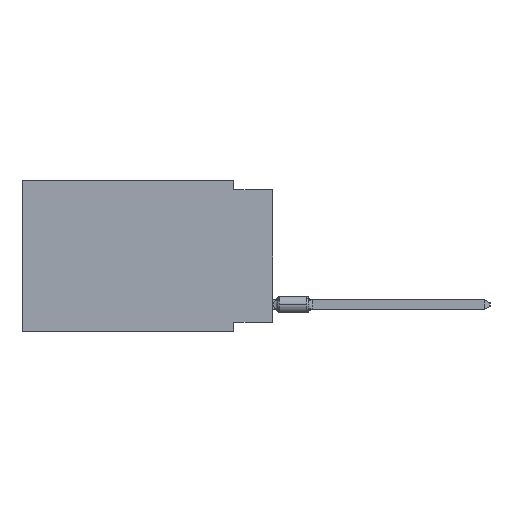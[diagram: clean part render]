
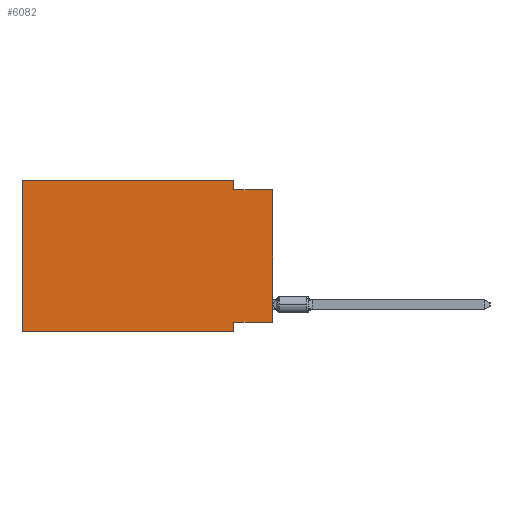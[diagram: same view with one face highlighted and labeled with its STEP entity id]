
A CAD part, left-side view. The second image highlights one B-rep face of the part: STEP entity #6082.
In plain terms, the highlighted planar face has unit normal (-1, 0, 0).
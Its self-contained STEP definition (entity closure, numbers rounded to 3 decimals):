
#603 = PLANE ( 'NONE',  #39979 ) ;
#1927 = LINE ( 'NONE', #6170, #13339 ) ;
#2528 = ORIENTED_EDGE ( 'NONE', *, *, #39677, .F. ) ;
#4096 = VECTOR ( 'NONE', #33010, 1000. ) ;
#4972 = LINE ( 'NONE', #29674, #46777 ) ;
#5116 = CARTESIAN_POINT ( 'NONE',  ( 0., 16.383, 0. ) ) ;
#5602 = ORIENTED_EDGE ( 'NONE', *, *, #21549, .F. ) ;
#6082 = ADVANCED_FACE ( 'NONE', ( #37013 ), #603, .F. ) ;
#6170 = CARTESIAN_POINT ( 'NONE',  ( 0., 0., -0.635 ) ) ;
#6790 = LINE ( 'NONE', #30448, #42864 ) ;
#8175 = EDGE_CURVE ( 'NONE', #9592, #27998, #50146, .T. ) ;
#9592 = VERTEX_POINT ( 'NONE', #29975 ) ;
#10128 = LINE ( 'NONE', #50221, #23848 ) ;
#10316 = DIRECTION ( 'NONE',  ( 0., -1., 0. ) ) ;
#10340 = VERTEX_POINT ( 'NONE', #44719 ) ;
#10588 = DIRECTION ( 'NONE',  ( 0., 0., -1. ) ) ;
#10955 = DIRECTION ( 'NONE',  ( 0., -1., 0. ) ) ;
#11740 = ORIENTED_EDGE ( 'NONE', *, *, #29530, .F. ) ;
#13339 = VECTOR ( 'NONE', #10955, 1000. ) ;
#13348 = DIRECTION ( 'NONE',  ( 0., 0., -1. ) ) ;
#13763 = CARTESIAN_POINT ( 'NONE',  ( 0., 0., -9.271 ) ) ;
#15226 = LINE ( 'NONE', #43377, #33491 ) ;
#16824 = DIRECTION ( 'NONE',  ( 1., 0., 0. ) ) ;
#17092 = EDGE_CURVE ( 'NONE', #48936, #21835, #1927, .T. ) ;
#17507 = VERTEX_POINT ( 'NONE', #50186 ) ;
#18624 = EDGE_CURVE ( 'NONE', #9592, #17507, #48688, .T. ) ;
#19208 = CARTESIAN_POINT ( 'NONE',  ( 0., 2.54, 0. ) ) ;
#20056 = VECTOR ( 'NONE', #10588, 1000. ) ;
#20294 = ORIENTED_EDGE ( 'NONE', *, *, #8175, .T. ) ;
#20651 = DIRECTION ( 'NONE',  ( 0., 0., -1. ) ) ;
#20991 = ORIENTED_EDGE ( 'NONE', *, *, #50594, .T. ) ;
#21549 = EDGE_CURVE ( 'NONE', #10340, #27998, #4972, .T. ) ;
#21835 = VERTEX_POINT ( 'NONE', #24021 ) ;
#22284 = CARTESIAN_POINT ( 'NONE',  ( 0., 2.54, 0. ) ) ;
#23266 = VECTOR ( 'NONE', #10316, 1000. ) ;
#23601 = CARTESIAN_POINT ( 'NONE',  ( 0., 2.54, -9.906 ) ) ;
#23848 = VECTOR ( 'NONE', #34835, 1000. ) ;
#24021 = CARTESIAN_POINT ( 'NONE',  ( 0., 0., -0.635 ) ) ;
#25937 = DIRECTION ( 'NONE',  ( 0., 0., 1. ) ) ;
#27998 = VERTEX_POINT ( 'NONE', #23601 ) ;
#29210 = ORIENTED_EDGE ( 'NONE', *, *, #18624, .F. ) ;
#29530 = EDGE_CURVE ( 'NONE', #30148, #10340, #10128, .T. ) ;
#29674 = CARTESIAN_POINT ( 'NONE',  ( 0., 2.54, -9.906 ) ) ;
#29975 = CARTESIAN_POINT ( 'NONE',  ( 0., 16.383, -9.906 ) ) ;
#30148 = VERTEX_POINT ( 'NONE', #13763 ) ;
#30448 = CARTESIAN_POINT ( 'NONE',  ( 0., 0., 0. ) ) ;
#30633 = DIRECTION ( 'NONE',  ( 0., -1., 0. ) ) ;
#33010 = DIRECTION ( 'NONE',  ( 0., 0., 1. ) ) ;
#33491 = VECTOR ( 'NONE', #30633, 1000. ) ;
#34232 = CARTESIAN_POINT ( 'NONE',  ( 0., 16.383, -9.906 ) ) ;
#34835 = DIRECTION ( 'NONE',  ( 0., 1., 0. ) ) ;
#36626 = VERTEX_POINT ( 'NONE', #19208 ) ;
#37013 = FACE_OUTER_BOUND ( 'NONE', #48849, .T. ) ;
#39677 = EDGE_CURVE ( 'NONE', #17507, #36626, #15226, .T. ) ;
#39979 = AXIS2_PLACEMENT_3D ( 'NONE', #5116, #16824, #13348 ) ;
#40397 = ORIENTED_EDGE ( 'NONE', *, *, #48397, .F. ) ;
#40735 = CARTESIAN_POINT ( 'NONE',  ( 0., 16.383, 0. ) ) ;
#42864 = VECTOR ( 'NONE', #25937, 1000. ) ;
#43377 = CARTESIAN_POINT ( 'NONE',  ( 0., 16.383, 0. ) ) ;
#44719 = CARTESIAN_POINT ( 'NONE',  ( 0., 2.54, -9.271 ) ) ;
#46777 = VECTOR ( 'NONE', #20651, 1000. ) ;
#47740 = ORIENTED_EDGE ( 'NONE', *, *, #17092, .F. ) ;
#48397 = EDGE_CURVE ( 'NONE', #36626, #48936, #50149, .T. ) ;
#48688 = LINE ( 'NONE', #40735, #4096 ) ;
#48849 = EDGE_LOOP ( 'NONE', ( #20991, #47740, #40397, #2528, #29210, #20294, #5602, #11740 ) ) ;
#48936 = VERTEX_POINT ( 'NONE', #49809 ) ;
#49809 = CARTESIAN_POINT ( 'NONE',  ( 0., 2.54, -0.635 ) ) ;
#50146 = LINE ( 'NONE', #34232, #23266 ) ;
#50149 = LINE ( 'NONE', #22284, #20056 ) ;
#50186 = CARTESIAN_POINT ( 'NONE',  ( 0., 16.383, 0. ) ) ;
#50221 = CARTESIAN_POINT ( 'NONE',  ( 0., 0., -9.271 ) ) ;
#50594 = EDGE_CURVE ( 'NONE', #30148, #21835, #6790, .T. ) ;
